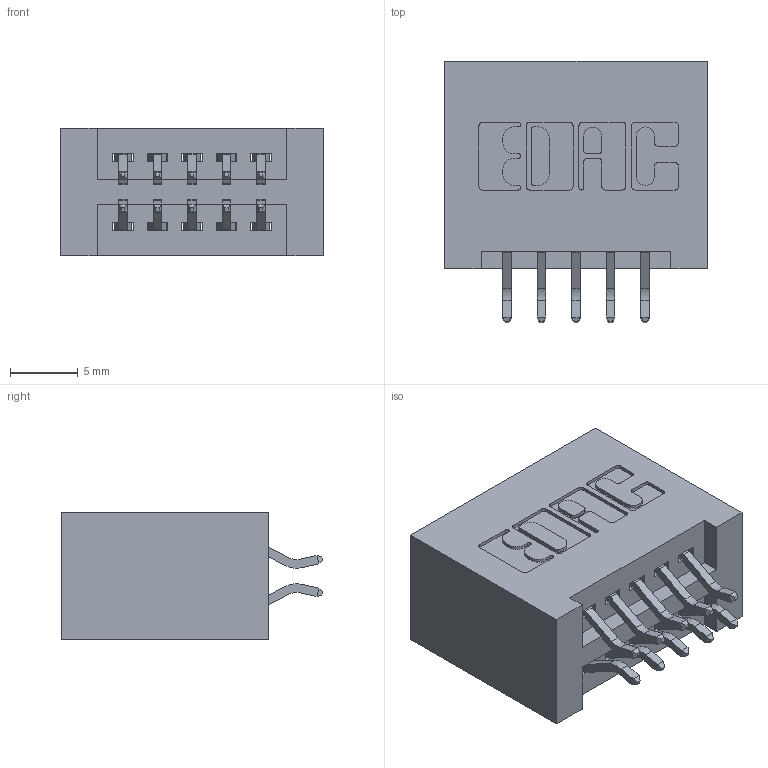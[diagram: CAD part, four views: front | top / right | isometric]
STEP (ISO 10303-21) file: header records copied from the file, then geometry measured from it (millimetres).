
FILE_DESCRIPTION (( 'STEP AP203' ), '1' );
FILE_NAME ('345-010-556-201.STEP', '2019-10-26T14:43:46', ( '' ), ( '' ), 'SwSTEP 2.0', 'SolidWorks 2016', '' );
FILE_SCHEMA (( 'CONFIG_CONTROL_DESIGN' ));
Length unit declared in the file: inch
Products named in the file (3): 345-292-001_556 Tail; 345-010-556-201; 345 Part_No Mounting Lugs
Assembly tree (11 placements, depth 2):
  345-010-556-201
    345 Part_No Mounting Lugs
    345-292-001_556 Tail  x10
Bounding box: 19.3 x 19.24 x 9.4 mm (x, y, z)
Volume: 2147.3 mm3; surface area: 2751.9 mm2
Topology: 11 solids, 11 shells, 678 faces, 1987 edges, 1310 vertices
Faces by surface type: plane 446, cylinder 232
Entity records: 8847 total; most frequent: CARTESIAN_POINT 1532, ORIENTED_EDGE 1454, DIRECTION 1379, EDGE_CURVE 727, LINE 575, VECTOR 575, VERTEX_POINT 482, AXIS2_PLACEMENT_3D 402
